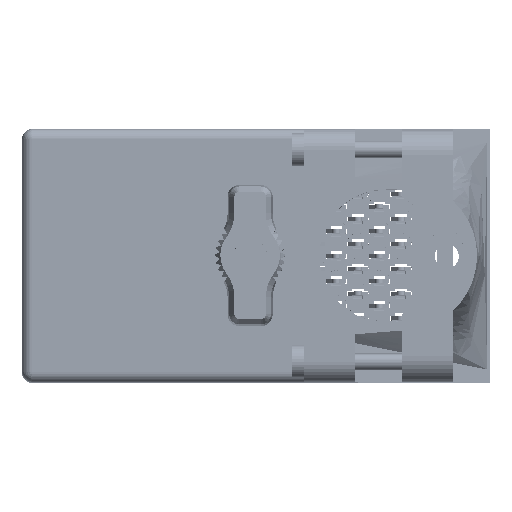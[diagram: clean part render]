
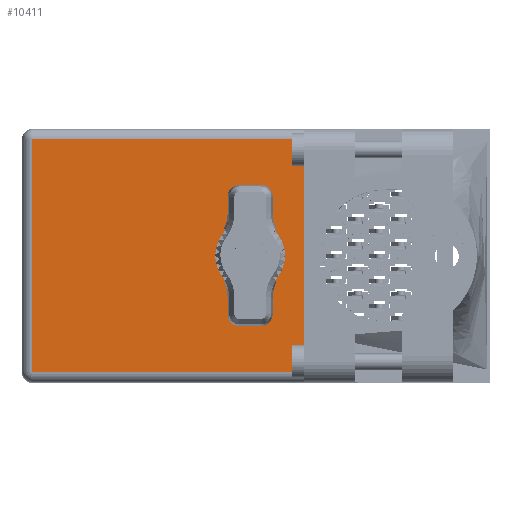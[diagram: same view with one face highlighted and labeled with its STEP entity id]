
A CAD part, top view. The second image highlights one B-rep face of the part: STEP entity #10411.
In plain terms, the highlighted face is planar.
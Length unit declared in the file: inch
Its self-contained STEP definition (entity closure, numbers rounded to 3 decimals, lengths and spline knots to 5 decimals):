
#1913 = ORIENTED_EDGE ( 'NONE', *, *, #13814, .T. ) ;
#7153 = DIRECTION ( 'NONE',  ( 0., 1., 0. ) ) ;
#7898 = ORIENTED_EDGE ( 'NONE', *, *, #53145, .F. ) ;
#9898 = CARTESIAN_POINT ( 'NONE',  ( -1.3155, 1.93, 0.703 ) ) ;
#9977 = VERTEX_POINT ( 'NONE', #89583 ) ;
#10218 = EDGE_CURVE ( 'NONE', #9977, #62713, #41122, .T. ) ;
#10411 = ADVANCED_FACE ( 'NONE', ( #38574, #11694 ), #28931, .T. ) ;
#11694 = FACE_BOUND ( 'NONE', #103028, .T. ) ;
#13814 = EDGE_CURVE ( 'NONE', #101068, #26435, #40424, .T. ) ;
#15407 = LINE ( 'NONE', #79751, #44903 ) ;
#18351 = EDGE_CURVE ( 'NONE', #62713, #9977, #98500, .T. ) ;
#20091 = CARTESIAN_POINT ( 'NONE',  ( 0., 1.93, 0.17 ) ) ;
#25272 = AXIS2_PLACEMENT_3D ( 'NONE', #61381, #86366, #37453 ) ;
#26435 = VERTEX_POINT ( 'NONE', #35655 ) ;
#27416 = ORIENTED_EDGE ( 'NONE', *, *, #57508, .T. ) ;
#28931 = PLANE ( 'NONE',  #25272 ) ;
#32394 = LINE ( 'NONE', #75357, #86011 ) ;
#32813 = VECTOR ( 'NONE', #49041, 39.37008 ) ;
#33889 = CARTESIAN_POINT ( 'NONE',  ( 0.3275, 1.93, -0.765 ) ) ;
#34738 = ORIENTED_EDGE ( 'NONE', *, *, #18351, .F. ) ;
#35655 = CARTESIAN_POINT ( 'NONE',  ( -1.3155, 1.93, -0.703 ) ) ;
#37453 = DIRECTION ( 'NONE',  ( -1., 0., 0. ) ) ;
#38574 = FACE_OUTER_BOUND ( 'NONE', #64021, .T. ) ;
#40424 = LINE ( 'NONE', #41808, #32813 ) ;
#41122 = CIRCLE ( 'NONE', #45789, 0.17 ) ;
#41808 = CARTESIAN_POINT ( 'NONE',  ( -1.3775, 1.93, -0.703 ) ) ;
#44903 = VECTOR ( 'NONE', #87264, 39.37008 ) ;
#45789 = AXIS2_PLACEMENT_3D ( 'NONE', #50605, #74818, #73779 ) ;
#48599 = ORIENTED_EDGE ( 'NONE', *, *, #10218, .F. ) ;
#49041 = DIRECTION ( 'NONE',  ( -1., 0., 0. ) ) ;
#50605 = CARTESIAN_POINT ( 'NONE',  ( 0., 1.93, 0. ) ) ;
#51126 = CARTESIAN_POINT ( 'NONE',  ( 0.3275, 1.93, -0.703 ) ) ;
#53145 = EDGE_CURVE ( 'NONE', #101068, #71146, #94081, .T. ) ;
#55272 = EDGE_CURVE ( 'NONE', #101869, #71146, #32394, .T. ) ;
#57508 = EDGE_CURVE ( 'NONE', #26435, #101869, #15407, .T. ) ;
#61381 = CARTESIAN_POINT ( 'NONE',  ( -1.3775, 1.93, -0.765 ) ) ;
#62713 = VERTEX_POINT ( 'NONE', #20091 ) ;
#64021 = EDGE_LOOP ( 'NONE', ( #27416, #67196, #7898, #1913 ) ) ;
#64267 = DIRECTION ( 'NONE',  ( 0., 0., 1. ) ) ;
#67196 = ORIENTED_EDGE ( 'NONE', *, *, #55272, .T. ) ;
#71146 = VERTEX_POINT ( 'NONE', #80538 ) ;
#72124 = CARTESIAN_POINT ( 'NONE',  ( 0., 1.93, 0. ) ) ;
#73779 = DIRECTION ( 'NONE',  ( 0., 0., 1. ) ) ;
#74818 = DIRECTION ( 'NONE',  ( 0., 1., 0. ) ) ;
#75357 = CARTESIAN_POINT ( 'NONE',  ( 0.3275, 1.93, 0.703 ) ) ;
#79651 = AXIS2_PLACEMENT_3D ( 'NONE', #72124, #7153, #64267 ) ;
#79751 = CARTESIAN_POINT ( 'NONE',  ( -1.3155, 1.93, -0.765 ) ) ;
#80538 = CARTESIAN_POINT ( 'NONE',  ( 0.3275, 1.93, 0.703 ) ) ;
#86011 = VECTOR ( 'NONE', #93959, 39.37008 ) ;
#86366 = DIRECTION ( 'NONE',  ( 0., 1., 0. ) ) ;
#87264 = DIRECTION ( 'NONE',  ( 0., 0., 1. ) ) ;
#89583 = CARTESIAN_POINT ( 'NONE',  ( 0., 1.93, -0.17 ) ) ;
#91001 = DIRECTION ( 'NONE',  ( 0., 0., 1. ) ) ;
#92858 = VECTOR ( 'NONE', #91001, 39.37008 ) ;
#93959 = DIRECTION ( 'NONE',  ( 1., 0., 0. ) ) ;
#94081 = LINE ( 'NONE', #33889, #92858 ) ;
#98500 = CIRCLE ( 'NONE', #79651, 0.17 ) ;
#101068 = VERTEX_POINT ( 'NONE', #51126 ) ;
#101869 = VERTEX_POINT ( 'NONE', #9898 ) ;
#103028 = EDGE_LOOP ( 'NONE', ( #34738, #48599 ) ) ;
